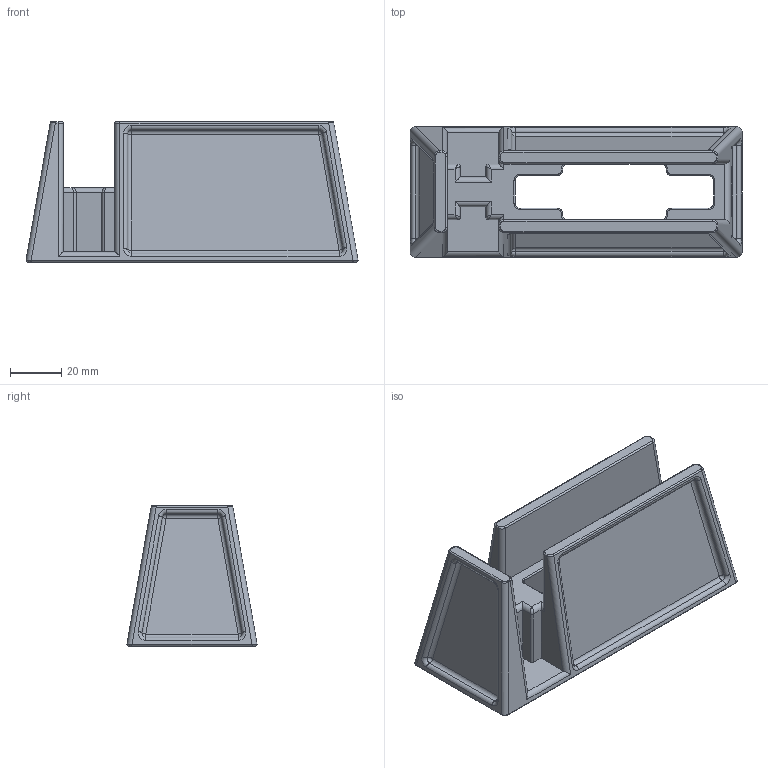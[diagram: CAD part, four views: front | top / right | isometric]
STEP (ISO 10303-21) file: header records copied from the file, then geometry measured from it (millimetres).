
FILE_DESCRIPTION(/* description */ (''),/* implementation_level */ '2;1');
FILE_NAME(/* name */ 'Glock Rear Sight Drift Block.step',/* time_stamp */ '2021-03-12T12:36:54-05:00',/* author */ (''),/* organization */ (''),/* preprocessor_version */ 'ST-DEVELOPER v18.1',/* originating_system */ 'Autodesk Translation Framework v9.10.0.1330',/* authorisation */ '');
FILE_SCHEMA (('AUTOMOTIVE_DESIGN { 1 0 10303 214 3 1 1 }'));
Length unit declared in the file: millimetre
Products named in the file (1): Glock Rear Sight Drift Block
Bounding box: 128.98 x 50.58 x 54.6 mm (x, y, z)
Volume: 105077.6 mm3; surface area: 37076.3 mm2
Topology: 1 solids, 1 shells, 354 faces, 888 edges, 540 vertices
Faces by surface type: bspline 140, cylinder 97, plane 83, torus 18, sphere 16
Entity records: 12089 total; most frequent: CARTESIAN_POINT 4556, ORIENTED_EDGE 1768, DIRECTION 1308, EDGE_CURVE 884, VERTEX_POINT 540, AXIS2_PLACEMENT_3D 441, LINE 426, VECTOR 426
